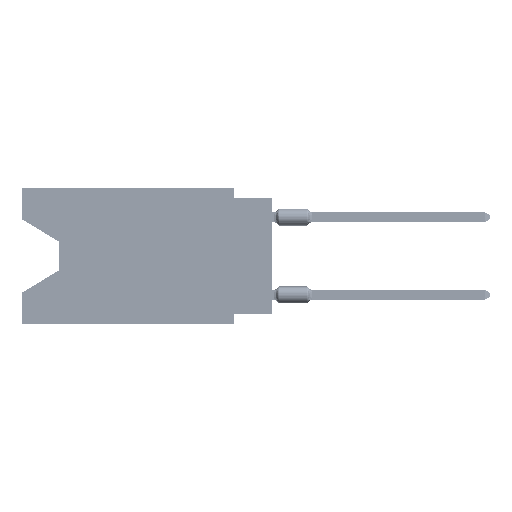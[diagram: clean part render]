
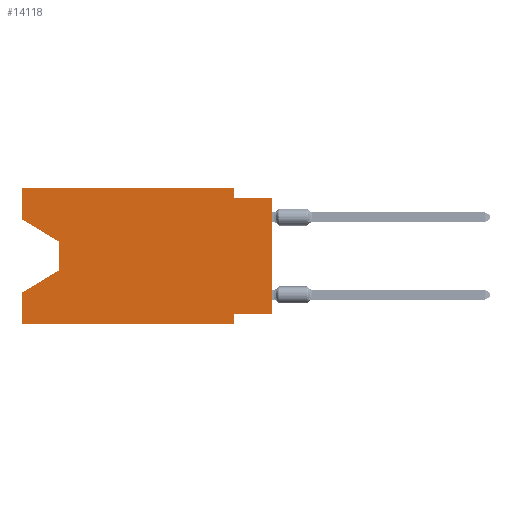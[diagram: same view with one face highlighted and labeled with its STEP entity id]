
A CAD part, left-side view. The second image highlights one B-rep face of the part: STEP entity #14118.
In plain terms, the highlighted planar face has unit normal (-1, 0, 0).
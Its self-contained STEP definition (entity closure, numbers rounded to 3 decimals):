
#344 = VERTEX_POINT ( 'NONE', #23864 ) ;
#2168 = CARTESIAN_POINT ( 'NONE',  ( 0., 16.383, -8.89 ) ) ;
#2314 = LINE ( 'NONE', #36280, #81953 ) ;
#5290 = EDGE_LOOP ( 'NONE', ( #37324, #73666, #21017, #69981, #58347, #74701, #20269, #46285, #82675, #82779, #15869, #31662 ) ) ;
#5562 = EDGE_CURVE ( 'NONE', #64133, #16876, #68733, .T. ) ;
#6954 = VERTEX_POINT ( 'NONE', #2168 ) ;
#7165 = VECTOR ( 'NONE', #15693, 1000. ) ;
#8967 = EDGE_CURVE ( 'NONE', #344, #60018, #22053, .T. ) ;
#9590 = CARTESIAN_POINT ( 'NONE',  ( 0., 13.97, -5.385 ) ) ;
#9957 = DIRECTION ( 'NONE',  ( 0., 0., -1. ) ) ;
#11331 = CARTESIAN_POINT ( 'NONE',  ( 0., 16.383, 0. ) ) ;
#12087 = CARTESIAN_POINT ( 'NONE',  ( 0., 0., -8.255 ) ) ;
#12133 = VECTOR ( 'NONE', #9957, 1000. ) ;
#13938 = VERTEX_POINT ( 'NONE', #68052 ) ;
#14118 = ADVANCED_FACE ( 'NONE', ( #77590 ), #71027, .F. ) ;
#14163 = CARTESIAN_POINT ( 'NONE',  ( 0., 2.54, -8.89 ) ) ;
#14215 = CARTESIAN_POINT ( 'NONE',  ( 0., 13.97, -3.505 ) ) ;
#14707 = VECTOR ( 'NONE', #70365, 1000. ) ;
#15277 = CARTESIAN_POINT ( 'NONE',  ( 0., 16.383, -2.038 ) ) ;
#15693 = DIRECTION ( 'NONE',  ( 0., -0.855, -0.519 ) ) ;
#15869 = ORIENTED_EDGE ( 'NONE', *, *, #5562, .F. ) ;
#16084 = VECTOR ( 'NONE', #81835, 1000. ) ;
#16876 = VERTEX_POINT ( 'NONE', #67159 ) ;
#16914 = VECTOR ( 'NONE', #65035, 1000. ) ;
#17685 = VERTEX_POINT ( 'NONE', #12087 ) ;
#20269 = ORIENTED_EDGE ( 'NONE', *, *, #57845, .F. ) ;
#21017 = ORIENTED_EDGE ( 'NONE', *, *, #59104, .T. ) ;
#22053 = LINE ( 'NONE', #34693, #52534 ) ;
#22443 = LINE ( 'NONE', #49008, #14707 ) ;
#22943 = CARTESIAN_POINT ( 'NONE',  ( 0., 0., 0. ) ) ;
#23496 = CARTESIAN_POINT ( 'NONE',  ( 0., 16.383, -2.038 ) ) ;
#23864 = CARTESIAN_POINT ( 'NONE',  ( 0., 2.54, -0.635 ) ) ;
#25325 = VECTOR ( 'NONE', #42704, 1000. ) ;
#27484 = DIRECTION ( 'NONE',  ( 0., 0., 1. ) ) ;
#28458 = DIRECTION ( 'NONE',  ( 0., 0., 1. ) ) ;
#29973 = CARTESIAN_POINT ( 'NONE',  ( 0., 13.97, -3.505 ) ) ;
#30342 = DIRECTION ( 'NONE',  ( 0., 0., 1. ) ) ;
#30512 = CARTESIAN_POINT ( 'NONE',  ( 0., 16.383, -8.89 ) ) ;
#31364 = DIRECTION ( 'NONE',  ( 1., 0., 0. ) ) ;
#31612 = VECTOR ( 'NONE', #73364, 1000. ) ;
#31662 = ORIENTED_EDGE ( 'NONE', *, *, #77476, .F. ) ;
#34693 = CARTESIAN_POINT ( 'NONE',  ( 0., 0., -0.635 ) ) ;
#36280 = CARTESIAN_POINT ( 'NONE',  ( 0., 16.383, 0. ) ) ;
#36617 = EDGE_CURVE ( 'NONE', #6954, #13938, #67147, .T. ) ;
#37324 = ORIENTED_EDGE ( 'NONE', *, *, #71227, .T. ) ;
#38437 = CARTESIAN_POINT ( 'NONE',  ( 0., 2.54, 0. ) ) ;
#38699 = VERTEX_POINT ( 'NONE', #14215 ) ;
#40907 = EDGE_CURVE ( 'NONE', #17685, #60018, #76131, .T. ) ;
#42704 = DIRECTION ( 'NONE',  ( 0., -1., 0. ) ) ;
#43459 = LINE ( 'NONE', #29973, #12133 ) ;
#45812 = CARTESIAN_POINT ( 'NONE',  ( 0., 2.54, -8.255 ) ) ;
#46000 = CARTESIAN_POINT ( 'NONE',  ( 0., 13.97, -5.385 ) ) ;
#46285 = ORIENTED_EDGE ( 'NONE', *, *, #40907, .T. ) ;
#46814 = EDGE_CURVE ( 'NONE', #83456, #49632, #22443, .T. ) ;
#49008 = CARTESIAN_POINT ( 'NONE',  ( 0., 2.54, -8.89 ) ) ;
#49632 = VERTEX_POINT ( 'NONE', #14163 ) ;
#50645 = VERTEX_POINT ( 'NONE', #23496 ) ;
#52534 = VECTOR ( 'NONE', #59994, 1000. ) ;
#53149 = VECTOR ( 'NONE', #30342, 1000. ) ;
#53284 = CARTESIAN_POINT ( 'NONE',  ( 0., 0., -8.255 ) ) ;
#57845 = EDGE_CURVE ( 'NONE', #17685, #83456, #72074, .T. ) ;
#57956 = DIRECTION ( 'NONE',  ( 0., 0., -1. ) ) ;
#58173 = VECTOR ( 'NONE', #78315, 1000. ) ;
#58347 = ORIENTED_EDGE ( 'NONE', *, *, #71844, .T. ) ;
#59104 = EDGE_CURVE ( 'NONE', #69476, #13938, #59112, .T. ) ;
#59112 = LINE ( 'NONE', #46000, #58173 ) ;
#59356 = LINE ( 'NONE', #38437, #16914 ) ;
#59474 = VECTOR ( 'NONE', #27484, 1000. ) ;
#59994 = DIRECTION ( 'NONE',  ( 0., -1., 0. ) ) ;
#60018 = VERTEX_POINT ( 'NONE', #70459 ) ;
#64133 = VERTEX_POINT ( 'NONE', #73748 ) ;
#65035 = DIRECTION ( 'NONE',  ( 0., 0., -1. ) ) ;
#67147 = LINE ( 'NONE', #67584, #59474 ) ;
#67159 = CARTESIAN_POINT ( 'NONE',  ( 0., 2.54, 0. ) ) ;
#67274 = AXIS2_PLACEMENT_3D ( 'NONE', #11331, #31364, #57956 ) ;
#67584 = CARTESIAN_POINT ( 'NONE',  ( 0., 16.383, 0. ) ) ;
#67586 = LINE ( 'NONE', #15277, #7165 ) ;
#68052 = CARTESIAN_POINT ( 'NONE',  ( 0., 16.383, -6.852 ) ) ;
#68733 = LINE ( 'NONE', #69586, #16084 ) ;
#69476 = VERTEX_POINT ( 'NONE', #9590 ) ;
#69586 = CARTESIAN_POINT ( 'NONE',  ( 0., 16.383, 0. ) ) ;
#69981 = ORIENTED_EDGE ( 'NONE', *, *, #36617, .F. ) ;
#70365 = DIRECTION ( 'NONE',  ( 0., 0., -1. ) ) ;
#70459 = CARTESIAN_POINT ( 'NONE',  ( 0., 0., -0.635 ) ) ;
#71027 = PLANE ( 'NONE',  #67274 ) ;
#71227 = EDGE_CURVE ( 'NONE', #50645, #38699, #67586, .T. ) ;
#71677 = EDGE_CURVE ( 'NONE', #16876, #344, #59356, .T. ) ;
#71844 = EDGE_CURVE ( 'NONE', #6954, #49632, #76734, .T. ) ;
#72074 = LINE ( 'NONE', #53284, #31612 ) ;
#73364 = DIRECTION ( 'NONE',  ( 0., 1., 0. ) ) ;
#73666 = ORIENTED_EDGE ( 'NONE', *, *, #75777, .T. ) ;
#73748 = CARTESIAN_POINT ( 'NONE',  ( 0., 16.383, 0. ) ) ;
#74701 = ORIENTED_EDGE ( 'NONE', *, *, #46814, .F. ) ;
#75777 = EDGE_CURVE ( 'NONE', #38699, #69476, #43459, .T. ) ;
#76131 = LINE ( 'NONE', #22943, #53149 ) ;
#76734 = LINE ( 'NONE', #30512, #25325 ) ;
#77476 = EDGE_CURVE ( 'NONE', #50645, #64133, #2314, .T. ) ;
#77590 = FACE_OUTER_BOUND ( 'NONE', #5290, .T. ) ;
#78315 = DIRECTION ( 'NONE',  ( 0., 0.855, -0.519 ) ) ;
#81835 = DIRECTION ( 'NONE',  ( 0., -1., 0. ) ) ;
#81953 = VECTOR ( 'NONE', #28458, 1000. ) ;
#82675 = ORIENTED_EDGE ( 'NONE', *, *, #8967, .F. ) ;
#82779 = ORIENTED_EDGE ( 'NONE', *, *, #71677, .F. ) ;
#83456 = VERTEX_POINT ( 'NONE', #45812 ) ;
